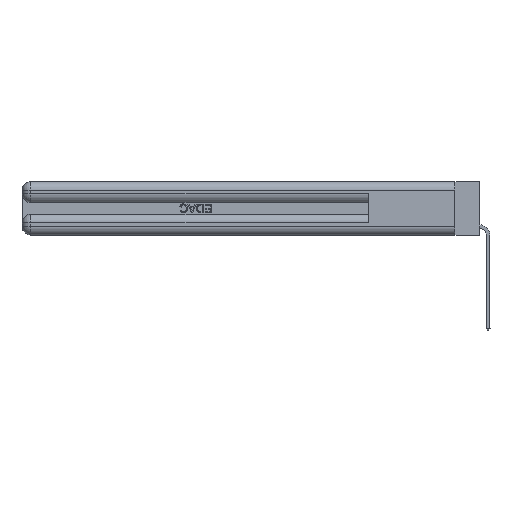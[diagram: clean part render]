
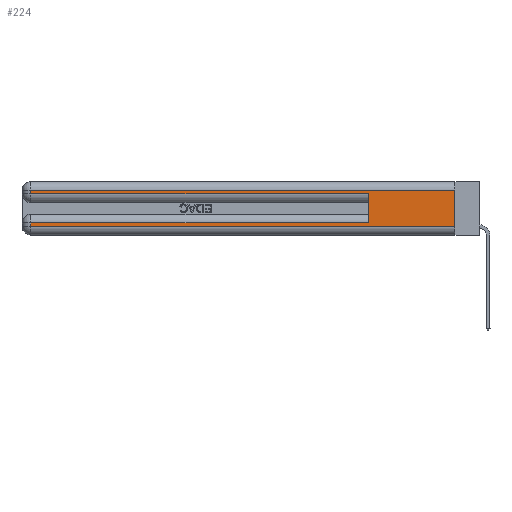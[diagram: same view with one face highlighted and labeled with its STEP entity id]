
A CAD part, left-side view. The second image highlights one B-rep face of the part: STEP entity #224.
In plain terms, the highlighted planar face has unit normal (-1, 0, 0).
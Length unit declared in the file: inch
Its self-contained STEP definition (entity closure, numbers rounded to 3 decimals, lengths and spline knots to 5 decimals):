
#224 = ADVANCED_FACE ( 'NONE', ( #9277 ), #9708, .F. ) ;
#961 = CARTESIAN_POINT ( 'NONE',  ( 0., 0., 0.285 ) ) ;
#995 = ORIENTED_EDGE ( 'NONE', *, *, #21899, .T. ) ;
#1011 = VERTEX_POINT ( 'NONE', #4751 ) ;
#2973 = DIRECTION ( 'NONE',  ( 0., -1., 0. ) ) ;
#3089 = VECTOR ( 'NONE', #20316, 39.37008 ) ;
#3138 = CARTESIAN_POINT ( 'NONE',  ( 0., 2.94, 0.085 ) ) ;
#3672 = ORIENTED_EDGE ( 'NONE', *, *, #6819, .F. ) ;
#4403 = VECTOR ( 'NONE', #6490, 39.37008 ) ;
#4751 = CARTESIAN_POINT ( 'NONE',  ( 0., 2.94, 0.285 ) ) ;
#5300 = CARTESIAN_POINT ( 'NONE',  ( 0., 2.94, 0.31 ) ) ;
#5350 = CARTESIAN_POINT ( 'NONE',  ( 0., 0.6, 0.285 ) ) ;
#5668 = EDGE_CURVE ( 'NONE', #23959, #9852, #6039, .T. ) ;
#6039 = LINE ( 'NONE', #13283, #15568 ) ;
#6400 = VERTEX_POINT ( 'NONE', #3138 ) ;
#6484 = VERTEX_POINT ( 'NONE', #5350 ) ;
#6490 = DIRECTION ( 'NONE',  ( 0., 0., -1. ) ) ;
#6702 = EDGE_CURVE ( 'NONE', #26121, #1011, #7558, .T. ) ;
#6819 = EDGE_CURVE ( 'NONE', #14157, #9852, #9755, .T. ) ;
#6847 = EDGE_CURVE ( 'NONE', #6400, #23959, #20539, .T. ) ;
#7558 = LINE ( 'NONE', #14096, #23070 ) ;
#7981 = EDGE_CURVE ( 'NONE', #22591, #6400, #25849, .T. ) ;
#8221 = EDGE_CURVE ( 'NONE', #1011, #6484, #15784, .T. ) ;
#8504 = CARTESIAN_POINT ( 'NONE',  ( 0., 2.94, 0.37 ) ) ;
#8705 = DIRECTION ( 'NONE',  ( 1., 0., 0. ) ) ;
#8779 = ORIENTED_EDGE ( 'NONE', *, *, #8221, .T. ) ;
#9277 = FACE_OUTER_BOUND ( 'NONE', #21714, .T. ) ;
#9554 = LINE ( 'NONE', #19260, #25056 ) ;
#9708 = PLANE ( 'NONE',  #13709 ) ;
#9739 = VECTOR ( 'NONE', #24441, 39.37008 ) ;
#9755 = LINE ( 'NONE', #12404, #4403 ) ;
#9852 = VERTEX_POINT ( 'NONE', #13538 ) ;
#10168 = CARTESIAN_POINT ( 'NONE',  ( 0., 0., 0.37 ) ) ;
#10282 = CARTESIAN_POINT ( 'NONE',  ( 0., 0., 0.085 ) ) ;
#10946 = ORIENTED_EDGE ( 'NONE', *, *, #5668, .T. ) ;
#10990 = VECTOR ( 'NONE', #2973, 39.37008 ) ;
#12404 = CARTESIAN_POINT ( 'NONE',  ( 0., 0., 0.37 ) ) ;
#13283 = CARTESIAN_POINT ( 'NONE',  ( 0., 0., 0.06 ) ) ;
#13538 = CARTESIAN_POINT ( 'NONE',  ( 0., 0., 0.06 ) ) ;
#13709 = AXIS2_PLACEMENT_3D ( 'NONE', #10168, #8705, #25953 ) ;
#14096 = CARTESIAN_POINT ( 'NONE',  ( 0., 2.94, 0.37 ) ) ;
#14157 = VERTEX_POINT ( 'NONE', #14465 ) ;
#14465 = CARTESIAN_POINT ( 'NONE',  ( 0., 0., 0.31 ) ) ;
#14542 = VECTOR ( 'NONE', #16684, 39.37008 ) ;
#14757 = ORIENTED_EDGE ( 'NONE', *, *, #7981, .T. ) ;
#15568 = VECTOR ( 'NONE', #17370, 39.37008 ) ;
#15607 = ORIENTED_EDGE ( 'NONE', *, *, #6847, .T. ) ;
#15784 = LINE ( 'NONE', #961, #10990 ) ;
#16684 = DIRECTION ( 'NONE',  ( 0., 0., -1. ) ) ;
#17370 = DIRECTION ( 'NONE',  ( 0., -1., 0. ) ) ;
#18169 = DIRECTION ( 'NONE',  ( 0., 0., -1. ) ) ;
#18300 = CARTESIAN_POINT ( 'NONE',  ( 0., 0., 0.31 ) ) ;
#18484 = ORIENTED_EDGE ( 'NONE', *, *, #18791, .F. ) ;
#18719 = CARTESIAN_POINT ( 'NONE',  ( 0., 0.6, 0.085 ) ) ;
#18791 = EDGE_CURVE ( 'NONE', #22591, #6484, #9554, .T. ) ;
#19242 = LINE ( 'NONE', #18300, #3089 ) ;
#19260 = CARTESIAN_POINT ( 'NONE',  ( 0., 0.6, 0.145 ) ) ;
#20316 = DIRECTION ( 'NONE',  ( 0., 1., 0. ) ) ;
#20539 = LINE ( 'NONE', #8504, #14542 ) ;
#21281 = DIRECTION ( 'NONE',  ( 0., 0., 1. ) ) ;
#21714 = EDGE_LOOP ( 'NONE', ( #3672, #995, #23630, #8779, #18484, #14757, #15607, #10946 ) ) ;
#21899 = EDGE_CURVE ( 'NONE', #14157, #26121, #19242, .T. ) ;
#22105 = CARTESIAN_POINT ( 'NONE',  ( 0., 2.94, 0.06 ) ) ;
#22591 = VERTEX_POINT ( 'NONE', #18719 ) ;
#23070 = VECTOR ( 'NONE', #18169, 39.37008 ) ;
#23630 = ORIENTED_EDGE ( 'NONE', *, *, #6702, .T. ) ;
#23959 = VERTEX_POINT ( 'NONE', #22105 ) ;
#24441 = DIRECTION ( 'NONE',  ( 0., 1., 0. ) ) ;
#25056 = VECTOR ( 'NONE', #21281, 39.37008 ) ;
#25849 = LINE ( 'NONE', #10282, #9739 ) ;
#25953 = DIRECTION ( 'NONE',  ( 0., 0., -1. ) ) ;
#26121 = VERTEX_POINT ( 'NONE', #5300 ) ;
